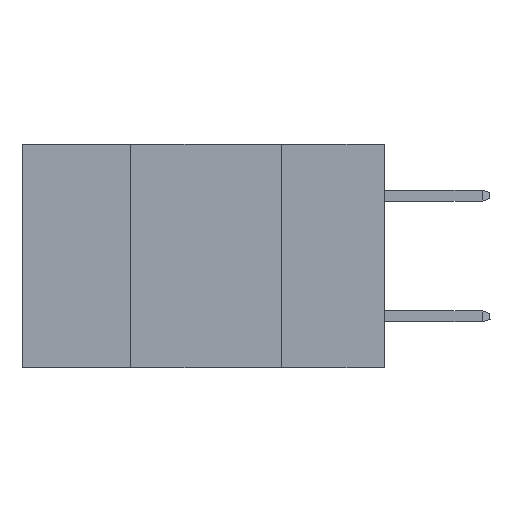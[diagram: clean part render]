
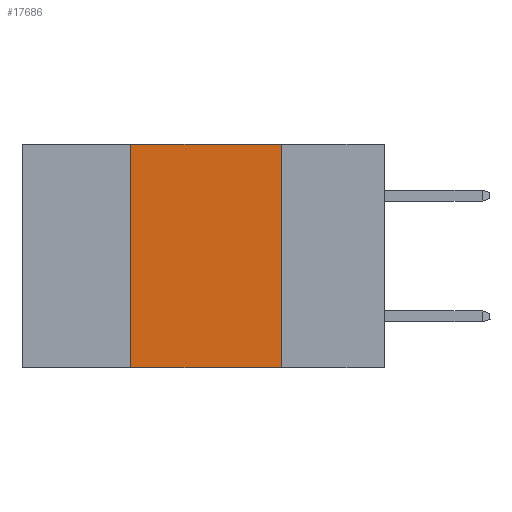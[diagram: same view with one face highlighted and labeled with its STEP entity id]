
A CAD part, left-side view. The second image highlights one B-rep face of the part: STEP entity #17686.
In plain terms, the highlighted planar face has unit normal (-1, 0, 0).
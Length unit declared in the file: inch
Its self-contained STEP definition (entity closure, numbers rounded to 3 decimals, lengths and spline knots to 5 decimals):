
#2510 = ORIENTED_EDGE ( 'NONE', *, *, #7728, .T. ) ;
#2587 = CARTESIAN_POINT ( 'NONE',  ( 0., 0.6, 0. ) ) ;
#3524 = LINE ( 'NONE', #8310, #24537 ) ;
#3838 = VERTEX_POINT ( 'NONE', #8617 ) ;
#4631 = DIRECTION ( 'NONE',  ( 0., -1., 0. ) ) ;
#5322 = CARTESIAN_POINT ( 'NONE',  ( 0., 0.6, -0.37 ) ) ;
#5496 = DIRECTION ( 'NONE',  ( 0., 0., -1. ) ) ;
#6160 = CARTESIAN_POINT ( 'NONE',  ( 0., 0.17, 0. ) ) ;
#6353 = DIRECTION ( 'NONE',  ( 0., 0., 1. ) ) ;
#7122 = VECTOR ( 'NONE', #4631, 39.37008 ) ;
#7386 = DIRECTION ( 'NONE',  ( 0., -1., 0. ) ) ;
#7728 = EDGE_CURVE ( 'NONE', #21719, #3838, #14592, .T. ) ;
#7951 = FACE_OUTER_BOUND ( 'NONE', #17796, .T. ) ;
#8310 = CARTESIAN_POINT ( 'NONE',  ( 0., 0.42, -0.37 ) ) ;
#8617 = CARTESIAN_POINT ( 'NONE',  ( 0., 0.17, -0.37 ) ) ;
#13621 = LINE ( 'NONE', #21828, #18371 ) ;
#14592 = LINE ( 'NONE', #5322, #24678 ) ;
#15348 = ORIENTED_EDGE ( 'NONE', *, *, #25918, .F. ) ;
#15748 = PLANE ( 'NONE',  #17277 ) ;
#16931 = ORIENTED_EDGE ( 'NONE', *, *, #23598, .F. ) ;
#17277 = AXIS2_PLACEMENT_3D ( 'NONE', #23769, #17793, #5496 ) ;
#17686 = ADVANCED_FACE ( 'NONE', ( #7951 ), #15748, .F. ) ;
#17693 = CARTESIAN_POINT ( 'NONE',  ( 0., 0.42, 0. ) ) ;
#17793 = DIRECTION ( 'NONE',  ( 1., 0., 0. ) ) ;
#17796 = EDGE_LOOP ( 'NONE', ( #18128, #16931, #15348, #2510 ) ) ;
#18128 = ORIENTED_EDGE ( 'NONE', *, *, #21241, .F. ) ;
#18371 = VECTOR ( 'NONE', #21747, 39.37008 ) ;
#20187 = VERTEX_POINT ( 'NONE', #6160 ) ;
#21241 = EDGE_CURVE ( 'NONE', #20187, #3838, #13621, .T. ) ;
#21719 = VERTEX_POINT ( 'NONE', #25006 ) ;
#21747 = DIRECTION ( 'NONE',  ( 0., 0., -1. ) ) ;
#21828 = CARTESIAN_POINT ( 'NONE',  ( 0., 0.17, -0.37 ) ) ;
#23379 = LINE ( 'NONE', #2587, #7122 ) ;
#23598 = EDGE_CURVE ( 'NONE', #24574, #20187, #23379, .T. ) ;
#23769 = CARTESIAN_POINT ( 'NONE',  ( 0., 0.6, 0. ) ) ;
#24537 = VECTOR ( 'NONE', #6353, 39.37008 ) ;
#24574 = VERTEX_POINT ( 'NONE', #17693 ) ;
#24678 = VECTOR ( 'NONE', #7386, 39.37008 ) ;
#25006 = CARTESIAN_POINT ( 'NONE',  ( 0., 0.42, -0.37 ) ) ;
#25918 = EDGE_CURVE ( 'NONE', #21719, #24574, #3524, .T. ) ;
